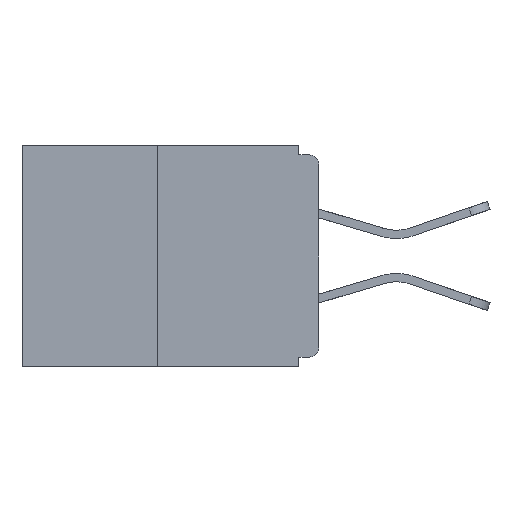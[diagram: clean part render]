
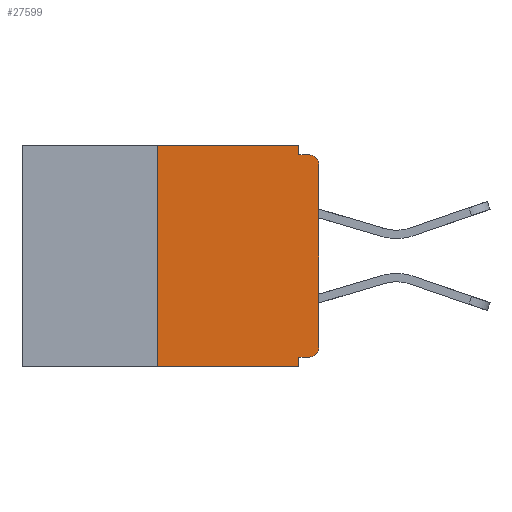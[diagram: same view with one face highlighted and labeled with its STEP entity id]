
A CAD part, left-side view. The second image highlights one B-rep face of the part: STEP entity #27599.
In plain terms, the highlighted planar face has unit normal (-1, 0, 0).
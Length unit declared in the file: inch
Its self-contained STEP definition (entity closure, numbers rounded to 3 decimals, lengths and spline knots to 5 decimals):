
#15 = CARTESIAN_POINT ( 'NONE',  ( 0., 0.46, 0. ) ) ;
#398 = CARTESIAN_POINT ( 'NONE',  ( 0., 0., 0. ) ) ;
#566 = CIRCLE ( 'NONE', #22339, 0.015 ) ;
#921 = LINE ( 'NONE', #9349, #2836 ) ;
#1057 = CARTESIAN_POINT ( 'NONE',  ( 0., 0.46, -0.343 ) ) ;
#1371 = VECTOR ( 'NONE', #7057, 39.37008 ) ;
#1870 = CARTESIAN_POINT ( 'NONE',  ( 0., 0., -0.313 ) ) ;
#1937 = CARTESIAN_POINT ( 'NONE',  ( 0., 0.015, -0.03 ) ) ;
#2047 = ORIENTED_EDGE ( 'NONE', *, *, #20006, .F. ) ;
#2084 = VERTEX_POINT ( 'NONE', #15940 ) ;
#2423 = DIRECTION ( 'NONE',  ( 0., 0., -1. ) ) ;
#2539 = DIRECTION ( 'NONE',  ( 0., 0., -1. ) ) ;
#2836 = VECTOR ( 'NONE', #29135, 39.37008 ) ;
#3066 = VECTOR ( 'NONE', #20818, 39.37008 ) ;
#4529 = VERTEX_POINT ( 'NONE', #6481 ) ;
#4782 = ORIENTED_EDGE ( 'NONE', *, *, #13846, .F. ) ;
#4953 = AXIS2_PLACEMENT_3D ( 'NONE', #1937, #6775, #21676 ) ;
#5319 = VERTEX_POINT ( 'NONE', #15105 ) ;
#5450 = ORIENTED_EDGE ( 'NONE', *, *, #10913, .F. ) ;
#6182 = VECTOR ( 'NONE', #18601, 39.37008 ) ;
#6449 = VECTOR ( 'NONE', #11021, 39.37008 ) ;
#6481 = CARTESIAN_POINT ( 'NONE',  ( 0., 0.25, -0.343 ) ) ;
#6614 = EDGE_CURVE ( 'NONE', #5319, #2084, #921, .T. ) ;
#6775 = DIRECTION ( 'NONE',  ( -1., 0., 0. ) ) ;
#6821 = CARTESIAN_POINT ( 'NONE',  ( 0., 0., -0.328 ) ) ;
#7057 = DIRECTION ( 'NONE',  ( 0., 0., -1. ) ) ;
#7542 = ORIENTED_EDGE ( 'NONE', *, *, #10817, .F. ) ;
#7662 = LINE ( 'NONE', #7970, #12691 ) ;
#7970 = CARTESIAN_POINT ( 'NONE',  ( 0., 0.25, 0. ) ) ;
#8266 = LINE ( 'NONE', #31747, #1371 ) ;
#8675 = LINE ( 'NONE', #6821, #16063 ) ;
#9349 = CARTESIAN_POINT ( 'NONE',  ( 0., 0.031, -0.343 ) ) ;
#9968 = FACE_OUTER_BOUND ( 'NONE', #11457, .T. ) ;
#10137 = ORIENTED_EDGE ( 'NONE', *, *, #10856, .T. ) ;
#10817 = EDGE_CURVE ( 'NONE', #12127, #16213, #8266, .T. ) ;
#10856 = EDGE_CURVE ( 'NONE', #26052, #22693, #566, .T. ) ;
#10913 = EDGE_CURVE ( 'NONE', #26052, #5319, #8675, .T. ) ;
#11021 = DIRECTION ( 'NONE',  ( 0., -1., 0. ) ) ;
#11457 = EDGE_LOOP ( 'NONE', ( #2047, #15611, #12498, #14042, #5450, #10137, #30041, #29449, #4782, #7542 ) ) ;
#12127 = VERTEX_POINT ( 'NONE', #28076 ) ;
#12498 = ORIENTED_EDGE ( 'NONE', *, *, #16127, .T. ) ;
#12691 = VECTOR ( 'NONE', #15243, 39.37008 ) ;
#13770 = CARTESIAN_POINT ( 'NONE',  ( 0., 0.46, 0. ) ) ;
#13846 = EDGE_CURVE ( 'NONE', #16213, #17631, #16514, .T. ) ;
#13936 = LINE ( 'NONE', #13770, #6182 ) ;
#14042 = ORIENTED_EDGE ( 'NONE', *, *, #6614, .F. ) ;
#14459 = CARTESIAN_POINT ( 'NONE',  ( 0., 0.015, -0.015 ) ) ;
#14616 = EDGE_CURVE ( 'NONE', #22693, #25521, #28624, .T. ) ;
#14713 = VERTEX_POINT ( 'NONE', #26268 ) ;
#14985 = DIRECTION ( 'NONE',  ( 1., 0., 0. ) ) ;
#15105 = CARTESIAN_POINT ( 'NONE',  ( 0., 0.031, -0.328 ) ) ;
#15243 = DIRECTION ( 'NONE',  ( 0., 0., 1. ) ) ;
#15395 = EDGE_CURVE ( 'NONE', #4529, #14713, #7662, .T. ) ;
#15611 = ORIENTED_EDGE ( 'NONE', *, *, #15395, .F. ) ;
#15832 = CARTESIAN_POINT ( 'NONE',  ( 0., 0.015, -0.328 ) ) ;
#15940 = CARTESIAN_POINT ( 'NONE',  ( 0., 0.031, -0.343 ) ) ;
#16063 = VECTOR ( 'NONE', #19040, 39.37008 ) ;
#16127 = EDGE_CURVE ( 'NONE', #4529, #2084, #20346, .T. ) ;
#16213 = VERTEX_POINT ( 'NONE', #28437 ) ;
#16514 = LINE ( 'NONE', #24626, #24619 ) ;
#17631 = VERTEX_POINT ( 'NONE', #14459 ) ;
#17917 = CARTESIAN_POINT ( 'NONE',  ( 0., 0., -0.03 ) ) ;
#18109 = AXIS2_PLACEMENT_3D ( 'NONE', #15, #14985, #2539 ) ;
#18601 = DIRECTION ( 'NONE',  ( 0., -1., 0. ) ) ;
#19040 = DIRECTION ( 'NONE',  ( 0., 1., 0. ) ) ;
#19696 = PLANE ( 'NONE',  #18109 ) ;
#20006 = EDGE_CURVE ( 'NONE', #14713, #12127, #13936, .T. ) ;
#20346 = LINE ( 'NONE', #1057, #6449 ) ;
#20818 = DIRECTION ( 'NONE',  ( 0., 0., 1. ) ) ;
#21676 = DIRECTION ( 'NONE',  ( 0., 0., -1. ) ) ;
#22203 = EDGE_CURVE ( 'NONE', #25521, #17631, #30451, .T. ) ;
#22339 = AXIS2_PLACEMENT_3D ( 'NONE', #27114, #24709, #2423 ) ;
#22693 = VERTEX_POINT ( 'NONE', #1870 ) ;
#24406 = DIRECTION ( 'NONE',  ( 0., -1., 0. ) ) ;
#24619 = VECTOR ( 'NONE', #24406, 39.37008 ) ;
#24626 = CARTESIAN_POINT ( 'NONE',  ( 0., 0., -0.015 ) ) ;
#24709 = DIRECTION ( 'NONE',  ( -1., 0., 0. ) ) ;
#25521 = VERTEX_POINT ( 'NONE', #17917 ) ;
#26052 = VERTEX_POINT ( 'NONE', #15832 ) ;
#26268 = CARTESIAN_POINT ( 'NONE',  ( 0., 0.25, 0. ) ) ;
#27114 = CARTESIAN_POINT ( 'NONE',  ( 0., 0.015, -0.313 ) ) ;
#27599 = ADVANCED_FACE ( 'NONE', ( #9968 ), #19696, .F. ) ;
#28076 = CARTESIAN_POINT ( 'NONE',  ( 0., 0.031, 0. ) ) ;
#28437 = CARTESIAN_POINT ( 'NONE',  ( 0., 0.031, -0.015 ) ) ;
#28624 = LINE ( 'NONE', #398, #3066 ) ;
#29135 = DIRECTION ( 'NONE',  ( 0., 0., -1. ) ) ;
#29449 = ORIENTED_EDGE ( 'NONE', *, *, #22203, .T. ) ;
#30041 = ORIENTED_EDGE ( 'NONE', *, *, #14616, .T. ) ;
#30451 = CIRCLE ( 'NONE', #4953, 0.015 ) ;
#31747 = CARTESIAN_POINT ( 'NONE',  ( 0., 0.031, 0. ) ) ;
